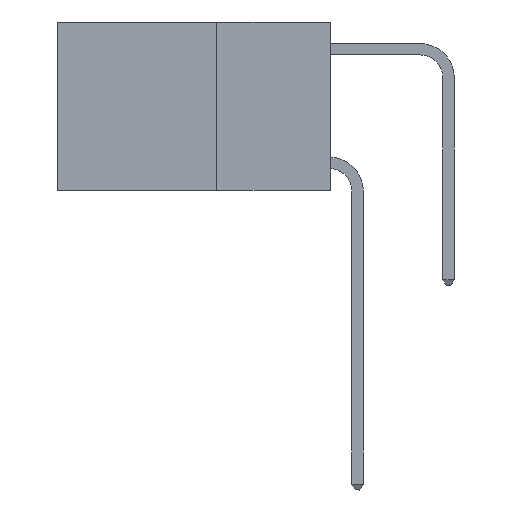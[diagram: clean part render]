
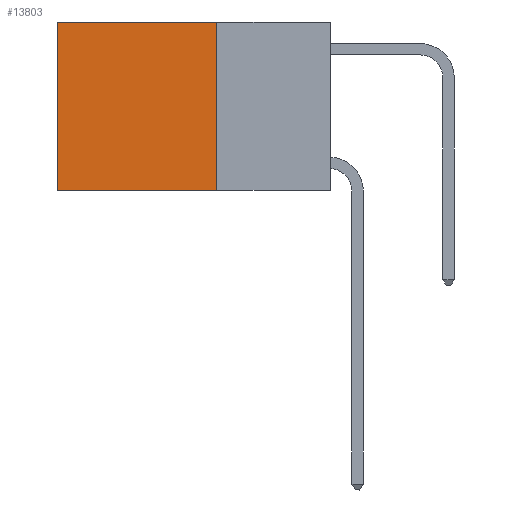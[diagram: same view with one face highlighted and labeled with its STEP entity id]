
A CAD part, left-side view. The second image highlights one B-rep face of the part: STEP entity #13803.
In plain terms, the highlighted planar face has unit normal (-1, 0, 0).
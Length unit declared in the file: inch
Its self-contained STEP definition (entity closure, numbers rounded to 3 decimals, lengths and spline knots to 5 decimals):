
#130 = CARTESIAN_POINT ( 'NONE',  ( 0.2625, 0.25, -0.37 ) ) ;
#421 = EDGE_CURVE ( 'NONE', #15594, #18808, #10856, .T. ) ;
#728 = EDGE_CURVE ( 'NONE', #13941, #19101, #12719, .T. ) ;
#1800 = AXIS2_PLACEMENT_3D ( 'NONE', #3981, #12923, #10011 ) ;
#2651 = EDGE_CURVE ( 'NONE', #19101, #18808, #18147, .T. ) ;
#3981 = CARTESIAN_POINT ( 'NONE',  ( 0.2625, 0.25, 0. ) ) ;
#4108 = LINE ( 'NONE', #7164, #15511 ) ;
#4361 = CARTESIAN_POINT ( 'NONE',  ( 0.2625, 0.25, 0. ) ) ;
#5656 = DIRECTION ( 'NONE',  ( 0., 0., -1. ) ) ;
#6309 = EDGE_CURVE ( 'NONE', #13941, #15594, #4108, .T. ) ;
#6999 = PLANE ( 'NONE',  #1800 ) ;
#7164 = CARTESIAN_POINT ( 'NONE',  ( 0.2625, 0.25, 0. ) ) ;
#7489 = ORIENTED_EDGE ( 'NONE', *, *, #6309, .F. ) ;
#7604 = ORIENTED_EDGE ( 'NONE', *, *, #728, .T. ) ;
#7828 = ORIENTED_EDGE ( 'NONE', *, *, #421, .F. ) ;
#7973 = CARTESIAN_POINT ( 'NONE',  ( 0.2625, 0.6, 0. ) ) ;
#8102 = CARTESIAN_POINT ( 'NONE',  ( 0.2625, 0.25, 0. ) ) ;
#9953 = VECTOR ( 'NONE', #14912, 39.37008 ) ;
#10011 = DIRECTION ( 'NONE',  ( 0., 0., -1. ) ) ;
#10176 = CARTESIAN_POINT ( 'NONE',  ( 0.2625, 0.6, 0. ) ) ;
#10856 = LINE ( 'NONE', #130, #9953 ) ;
#11918 = DIRECTION ( 'NONE',  ( 0., 1., 0. ) ) ;
#12403 = ORIENTED_EDGE ( 'NONE', *, *, #2651, .T. ) ;
#12719 = LINE ( 'NONE', #8102, #17070 ) ;
#12923 = DIRECTION ( 'NONE',  ( 1., 0., 0. ) ) ;
#13803 = ADVANCED_FACE ( 'NONE', ( #18486 ), #6999, .F. ) ;
#13941 = VERTEX_POINT ( 'NONE', #4361 ) ;
#14263 = VECTOR ( 'NONE', #17573, 39.37008 ) ;
#14912 = DIRECTION ( 'NONE',  ( 0., 1., 0. ) ) ;
#15434 = EDGE_LOOP ( 'NONE', ( #12403, #7828, #7489, #7604 ) ) ;
#15511 = VECTOR ( 'NONE', #5656, 39.37008 ) ;
#15594 = VERTEX_POINT ( 'NONE', #17654 ) ;
#17070 = VECTOR ( 'NONE', #11918, 39.37008 ) ;
#17573 = DIRECTION ( 'NONE',  ( 0., 0., -1. ) ) ;
#17654 = CARTESIAN_POINT ( 'NONE',  ( 0.2625, 0.25, -0.37 ) ) ;
#18147 = LINE ( 'NONE', #10176, #14263 ) ;
#18486 = FACE_OUTER_BOUND ( 'NONE', #15434, .T. ) ;
#18808 = VERTEX_POINT ( 'NONE', #19175 ) ;
#19101 = VERTEX_POINT ( 'NONE', #7973 ) ;
#19175 = CARTESIAN_POINT ( 'NONE',  ( 0.2625, 0.6, -0.37 ) ) ;
